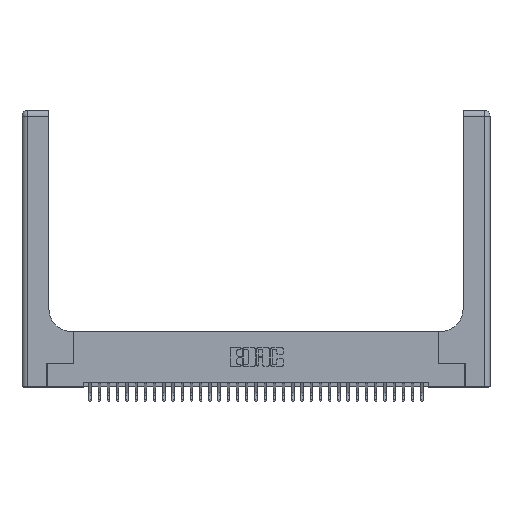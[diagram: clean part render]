
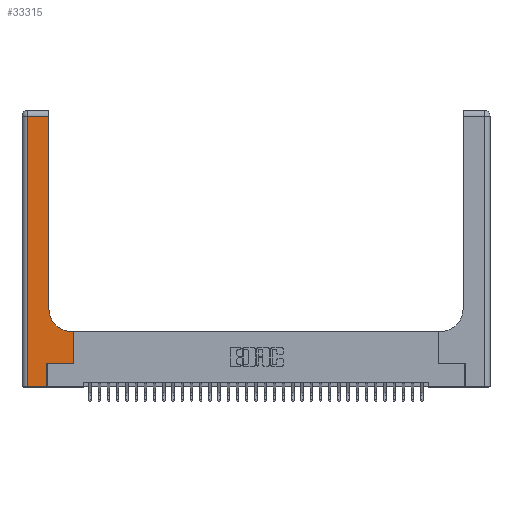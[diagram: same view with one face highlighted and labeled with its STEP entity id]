
A CAD part, top view. The second image highlights one B-rep face of the part: STEP entity #33315.
In plain terms, the highlighted planar face has unit normal (0, 0, 1).
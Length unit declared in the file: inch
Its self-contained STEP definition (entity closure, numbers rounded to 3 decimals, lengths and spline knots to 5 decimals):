
#342 = LINE ( 'NONE', #29626, #33930 ) ;
#823 = LINE ( 'NONE', #1526, #23401 ) ;
#1435 = ORIENTED_EDGE ( 'NONE', *, *, #9987, .T. ) ;
#1526 = CARTESIAN_POINT ( 'NONE',  ( 0., 0., 0.37 ) ) ;
#2981 = VERTEX_POINT ( 'NONE', #11629 ) ;
#3872 = DIRECTION ( 'NONE',  ( 1., 0., 0. ) ) ;
#4042 = VERTEX_POINT ( 'NONE', #26655 ) ;
#4654 = CARTESIAN_POINT ( 'NONE',  ( 0.5415, 0.6, 0.37 ) ) ;
#4687 = DIRECTION ( 'NONE',  ( -1., 0., 0. ) ) ;
#5209 = ORIENTED_EDGE ( 'NONE', *, *, #13874, .T. ) ;
#6351 = VERTEX_POINT ( 'NONE', #4654 ) ;
#6789 = VERTEX_POINT ( 'NONE', #21561 ) ;
#7447 = CARTESIAN_POINT ( 'NONE',  ( 0.2915, 0.6, 0.37 ) ) ;
#7930 = CIRCLE ( 'NONE', #15976, 0.25 ) ;
#8093 = DIRECTION ( 'NONE',  ( 1., 0., 0. ) ) ;
#8554 = VERTEX_POINT ( 'NONE', #15516 ) ;
#9392 = VECTOR ( 'NONE', #4687, 39.37008 ) ;
#9818 = PLANE ( 'NONE',  #12980 ) ;
#9987 = EDGE_CURVE ( 'NONE', #20573, #2981, #32520, .T. ) ;
#10009 = VECTOR ( 'NONE', #8093, 39.37008 ) ;
#10630 = DIRECTION ( 'NONE',  ( 0., -1., 0. ) ) ;
#10709 = EDGE_CURVE ( 'NONE', #13998, #20573, #823, .T. ) ;
#10933 = EDGE_CURVE ( 'NONE', #11703, #6351, #28497, .T. ) ;
#11629 = CARTESIAN_POINT ( 'NONE',  ( 0.269, 0.25, 0.37 ) ) ;
#11703 = VERTEX_POINT ( 'NONE', #21278 ) ;
#12276 = FACE_OUTER_BOUND ( 'NONE', #23076, .T. ) ;
#12285 = ORIENTED_EDGE ( 'NONE', *, *, #17243, .T. ) ;
#12980 = AXIS2_PLACEMENT_3D ( 'NONE', #25826, #15254, #33886 ) ;
#13310 = DIRECTION ( 'NONE',  ( 0., 1., 0. ) ) ;
#13874 = EDGE_CURVE ( 'NONE', #6351, #8554, #7930, .T. ) ;
#13998 = VERTEX_POINT ( 'NONE', #25331 ) ;
#15254 = DIRECTION ( 'NONE',  ( 0., 0., -1. ) ) ;
#15516 = CARTESIAN_POINT ( 'NONE',  ( 0.2915, 0.85, 0.37 ) ) ;
#15598 = EDGE_CURVE ( 'NONE', #4042, #11703, #34128, .T. ) ;
#15795 = DIRECTION ( 'NONE',  ( 0., 0., -1. ) ) ;
#15916 = EDGE_CURVE ( 'NONE', #6789, #30919, #24333, .T. ) ;
#15976 = AXIS2_PLACEMENT_3D ( 'NONE', #24887, #15795, #34545 ) ;
#16583 = CARTESIAN_POINT ( 'NONE',  ( 0., 2.94, 0.37 ) ) ;
#17093 = VECTOR ( 'NONE', #22258, 39.37008 ) ;
#17197 = LINE ( 'NONE', #21838, #10009 ) ;
#17243 = EDGE_CURVE ( 'NONE', #8554, #6789, #22241, .T. ) ;
#18681 = CARTESIAN_POINT ( 'NONE',  ( 0.2915, 3., 0.37 ) ) ;
#18920 = DIRECTION ( 'NONE',  ( 0., 1., 0. ) ) ;
#19250 = VECTOR ( 'NONE', #32073, 39.37008 ) ;
#20573 = VERTEX_POINT ( 'NONE', #26420 ) ;
#21003 = CARTESIAN_POINT ( 'NONE',  ( 0.269, 0., 0.37 ) ) ;
#21023 = ORIENTED_EDGE ( 'NONE', *, *, #15598, .T. ) ;
#21278 = CARTESIAN_POINT ( 'NONE',  ( 0.5585, 0.6, 0.37 ) ) ;
#21561 = CARTESIAN_POINT ( 'NONE',  ( 0.2915, 2.94, 0.37 ) ) ;
#21838 = CARTESIAN_POINT ( 'NONE',  ( 0.269, 0.25, 0.37 ) ) ;
#22241 = LINE ( 'NONE', #18681, #28630 ) ;
#22258 = DIRECTION ( 'NONE',  ( -1., 0., 0. ) ) ;
#23076 = EDGE_LOOP ( 'NONE', ( #12285, #33324, #32207, #34117, #1435, #24840, #21023, #32039, #5209 ) ) ;
#23401 = VECTOR ( 'NONE', #3872, 39.37008 ) ;
#24333 = LINE ( 'NONE', #16583, #17093 ) ;
#24840 = ORIENTED_EDGE ( 'NONE', *, *, #25992, .T. ) ;
#24887 = CARTESIAN_POINT ( 'NONE',  ( 0.5415, 0.85, 0.37 ) ) ;
#25331 = CARTESIAN_POINT ( 'NONE',  ( 0.06, 0., 0.37 ) ) ;
#25826 = CARTESIAN_POINT ( 'NONE',  ( 0., 3., 0.37 ) ) ;
#25992 = EDGE_CURVE ( 'NONE', #2981, #4042, #17197, .T. ) ;
#26233 = CARTESIAN_POINT ( 'NONE',  ( 0.5585, 0.25, 0.37 ) ) ;
#26420 = CARTESIAN_POINT ( 'NONE',  ( 0.269, 0., 0.37 ) ) ;
#26655 = CARTESIAN_POINT ( 'NONE',  ( 0.5585, 0.25, 0.37 ) ) ;
#28497 = LINE ( 'NONE', #7447, #9392 ) ;
#28630 = VECTOR ( 'NONE', #18920, 39.37008 ) ;
#29626 = CARTESIAN_POINT ( 'NONE',  ( 0.06, 3., 0.37 ) ) ;
#30518 = CARTESIAN_POINT ( 'NONE',  ( 0.06, 2.94, 0.37 ) ) ;
#30919 = VERTEX_POINT ( 'NONE', #30518 ) ;
#32039 = ORIENTED_EDGE ( 'NONE', *, *, #10933, .T. ) ;
#32073 = DIRECTION ( 'NONE',  ( 0., 1., 0. ) ) ;
#32207 = ORIENTED_EDGE ( 'NONE', *, *, #33508, .T. ) ;
#32520 = LINE ( 'NONE', #21003, #34152 ) ;
#33315 = ADVANCED_FACE ( 'NONE', ( #12276 ), #9818, .F. ) ;
#33324 = ORIENTED_EDGE ( 'NONE', *, *, #15916, .T. ) ;
#33508 = EDGE_CURVE ( 'NONE', #30919, #13998, #342, .T. ) ;
#33886 = DIRECTION ( 'NONE',  ( -1., 0., 0. ) ) ;
#33930 = VECTOR ( 'NONE', #10630, 39.37008 ) ;
#34117 = ORIENTED_EDGE ( 'NONE', *, *, #10709, .T. ) ;
#34128 = LINE ( 'NONE', #26233, #19250 ) ;
#34152 = VECTOR ( 'NONE', #13310, 39.37008 ) ;
#34545 = DIRECTION ( 'NONE',  ( 1., 0., 0. ) ) ;
